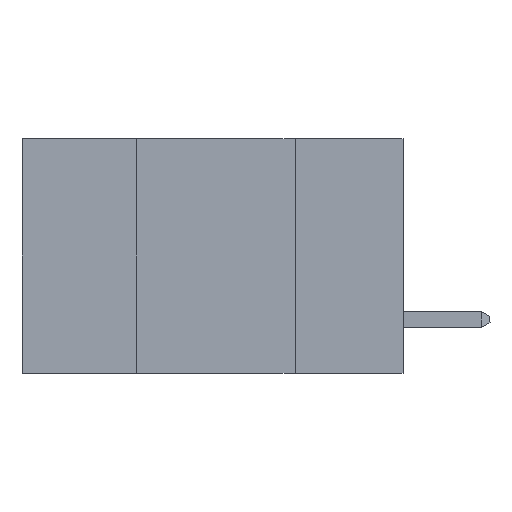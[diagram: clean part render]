
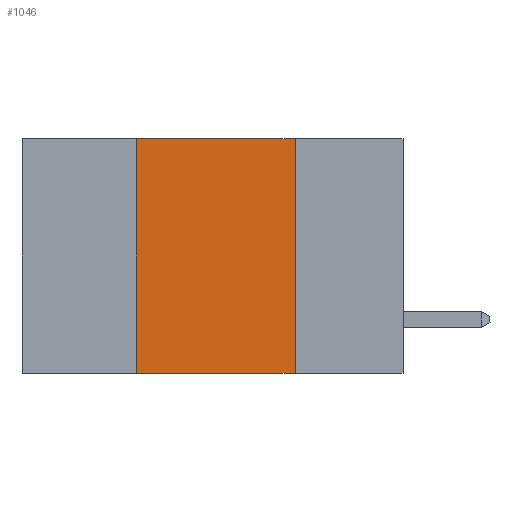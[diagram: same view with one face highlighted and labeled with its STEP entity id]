
A CAD part, left-side view. The second image highlights one B-rep face of the part: STEP entity #1046.
In plain terms, the highlighted planar face has unit normal (-1, 0, 0).
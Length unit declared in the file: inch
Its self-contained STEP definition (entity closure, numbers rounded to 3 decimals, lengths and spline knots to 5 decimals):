
#931 = ORIENTED_EDGE ( 'NONE', *, *, #8691, .F. ) ;
#1045 = ORIENTED_EDGE ( 'NONE', *, *, #6507, .T. ) ;
#1046 = ADVANCED_FACE ( 'NONE', ( #4375 ), #7057, .F. ) ;
#1214 = VECTOR ( 'NONE', #7008, 39.37008 ) ;
#2373 = CARTESIAN_POINT ( 'NONE',  ( 0., 0.42, 0. ) ) ;
#2381 = ORIENTED_EDGE ( 'NONE', *, *, #9508, .F. ) ;
#2439 = VERTEX_POINT ( 'NONE', #6993 ) ;
#3288 = ORIENTED_EDGE ( 'NONE', *, *, #5300, .F. ) ;
#3327 = AXIS2_PLACEMENT_3D ( 'NONE', #7904, #5661, #7495 ) ;
#4375 = FACE_OUTER_BOUND ( 'NONE', #4481, .T. ) ;
#4481 = EDGE_LOOP ( 'NONE', ( #2381, #3288, #931, #1045 ) ) ;
#4545 = VERTEX_POINT ( 'NONE', #8931 ) ;
#4853 = LINE ( 'NONE', #7084, #8465 ) ;
#4891 = VERTEX_POINT ( 'NONE', #7399 ) ;
#5300 = EDGE_CURVE ( 'NONE', #4891, #4545, #7296, .T. ) ;
#5581 = DIRECTION ( 'NONE',  ( 0., -1., 0. ) ) ;
#5661 = DIRECTION ( 'NONE',  ( 1., 0., 0. ) ) ;
#5716 = CARTESIAN_POINT ( 'NONE',  ( 0., 0.6, 0. ) ) ;
#6292 = CARTESIAN_POINT ( 'NONE',  ( 0., 0.17, 0. ) ) ;
#6507 = EDGE_CURVE ( 'NONE', #8770, #2439, #4853, .T. ) ;
#6993 = CARTESIAN_POINT ( 'NONE',  ( 0., 0.17, -0.37 ) ) ;
#7008 = DIRECTION ( 'NONE',  ( 0., 0., -1. ) ) ;
#7057 = PLANE ( 'NONE',  #3327 ) ;
#7066 = VECTOR ( 'NONE', #5581, 39.37008 ) ;
#7084 = CARTESIAN_POINT ( 'NONE',  ( 0., 0.6, -0.37 ) ) ;
#7296 = LINE ( 'NONE', #5716, #7066 ) ;
#7399 = CARTESIAN_POINT ( 'NONE',  ( 0., 0.42, 0. ) ) ;
#7495 = DIRECTION ( 'NONE',  ( 0., 0., -1. ) ) ;
#7524 = LINE ( 'NONE', #6292, #1214 ) ;
#7770 = DIRECTION ( 'NONE',  ( 0., -1., 0. ) ) ;
#7772 = CARTESIAN_POINT ( 'NONE',  ( 0., 0.42, -0.37 ) ) ;
#7904 = CARTESIAN_POINT ( 'NONE',  ( 0., 0.6, 0. ) ) ;
#8465 = VECTOR ( 'NONE', #7770, 39.37008 ) ;
#8542 = VECTOR ( 'NONE', #9123, 39.37008 ) ;
#8691 = EDGE_CURVE ( 'NONE', #8770, #4891, #8989, .T. ) ;
#8770 = VERTEX_POINT ( 'NONE', #7772 ) ;
#8931 = CARTESIAN_POINT ( 'NONE',  ( 0., 0.17, 0. ) ) ;
#8989 = LINE ( 'NONE', #2373, #8542 ) ;
#9123 = DIRECTION ( 'NONE',  ( 0., 0., 1. ) ) ;
#9508 = EDGE_CURVE ( 'NONE', #4545, #2439, #7524, .T. ) ;
